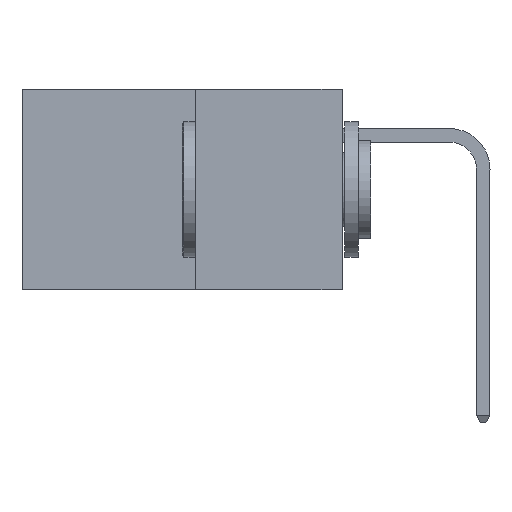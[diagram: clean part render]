
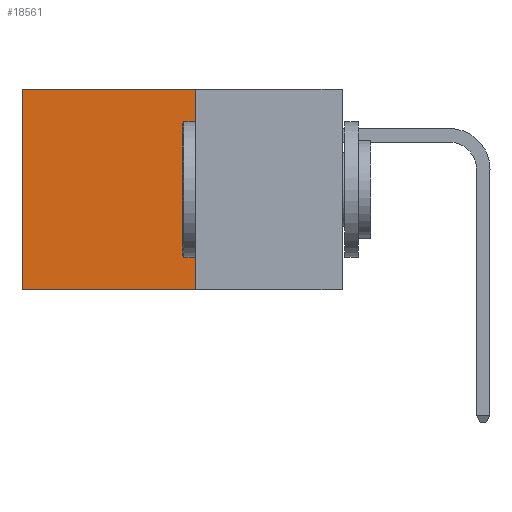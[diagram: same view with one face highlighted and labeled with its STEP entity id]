
A CAD part, left-side view. The second image highlights one B-rep face of the part: STEP entity #18561.
In plain terms, the highlighted planar face has unit normal (-1, 0, 0).
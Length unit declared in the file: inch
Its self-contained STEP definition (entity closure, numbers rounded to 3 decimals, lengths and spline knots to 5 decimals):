
#955 = CARTESIAN_POINT ( 'NONE',  ( 0.277, 0.27, -0.37 ) ) ;
#1011 = EDGE_CURVE ( 'NONE', #14323, #21479, #12872, .T. ) ;
#2017 = AXIS2_PLACEMENT_3D ( 'NONE', #955, #3149, #18640 ) ;
#3149 = DIRECTION ( 'NONE',  ( 1., 0., 0. ) ) ;
#3439 = LINE ( 'NONE', #17154, #25607 ) ;
#3848 = VECTOR ( 'NONE', #22043, 39.37008 ) ;
#4318 = CARTESIAN_POINT ( 'NONE',  ( 0.277, 0.27, 0. ) ) ;
#6037 = CARTESIAN_POINT ( 'NONE',  ( 0.277, 0.27, 0. ) ) ;
#6863 = ORIENTED_EDGE ( 'NONE', *, *, #8650, .T. ) ;
#7842 = CARTESIAN_POINT ( 'NONE',  ( 0.277, 0.27, -0.37 ) ) ;
#8016 = ORIENTED_EDGE ( 'NONE', *, *, #1011, .F. ) ;
#8650 = EDGE_CURVE ( 'NONE', #12445, #8855, #3439, .T. ) ;
#8855 = VERTEX_POINT ( 'NONE', #22240 ) ;
#8913 = CARTESIAN_POINT ( 'NONE',  ( 0.277, 0.59, 0. ) ) ;
#9574 = DIRECTION ( 'NONE',  ( 0., 0., -1. ) ) ;
#9640 = CARTESIAN_POINT ( 'NONE',  ( 0.277, 0.27, -0.37 ) ) ;
#12445 = VERTEX_POINT ( 'NONE', #8913 ) ;
#12699 = ORIENTED_EDGE ( 'NONE', *, *, #15476, .T. ) ;
#12872 = LINE ( 'NONE', #9640, #19532 ) ;
#14122 = PLANE ( 'NONE',  #2017 ) ;
#14323 = VERTEX_POINT ( 'NONE', #6037 ) ;
#14595 = EDGE_CURVE ( 'NONE', #21479, #8855, #28202, .T. ) ;
#15476 = EDGE_CURVE ( 'NONE', #14323, #12445, #21538, .T. ) ;
#16106 = ORIENTED_EDGE ( 'NONE', *, *, #14595, .F. ) ;
#16360 = VECTOR ( 'NONE', #20196, 39.37008 ) ;
#17154 = CARTESIAN_POINT ( 'NONE',  ( 0.277, 0.59, -0.37 ) ) ;
#18561 = ADVANCED_FACE ( 'NONE', ( #21733 ), #14122, .F. ) ;
#18640 = DIRECTION ( 'NONE',  ( 0., 0., -1. ) ) ;
#19532 = VECTOR ( 'NONE', #9574, 39.37008 ) ;
#20196 = DIRECTION ( 'NONE',  ( 0., 1., 0. ) ) ;
#21479 = VERTEX_POINT ( 'NONE', #7842 ) ;
#21538 = LINE ( 'NONE', #4318, #3848 ) ;
#21733 = FACE_OUTER_BOUND ( 'NONE', #27766, .T. ) ;
#22043 = DIRECTION ( 'NONE',  ( 0., 1., 0. ) ) ;
#22240 = CARTESIAN_POINT ( 'NONE',  ( 0.277, 0.59, -0.37 ) ) ;
#25607 = VECTOR ( 'NONE', #28534, 39.37008 ) ;
#26768 = CARTESIAN_POINT ( 'NONE',  ( 0.277, 0.27, -0.37 ) ) ;
#27766 = EDGE_LOOP ( 'NONE', ( #6863, #16106, #8016, #12699 ) ) ;
#28202 = LINE ( 'NONE', #26768, #16360 ) ;
#28534 = DIRECTION ( 'NONE',  ( 0., 0., -1. ) ) ;
